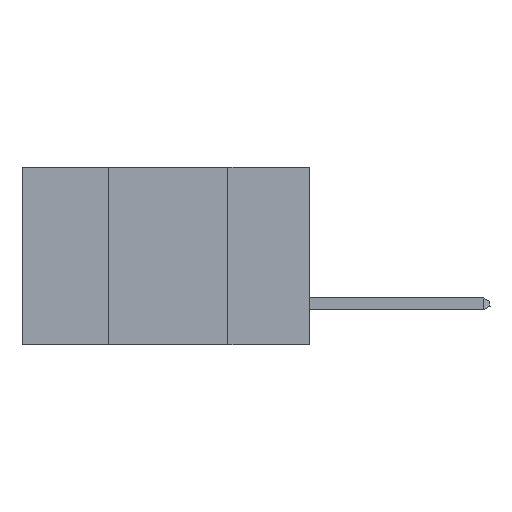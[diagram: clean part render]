
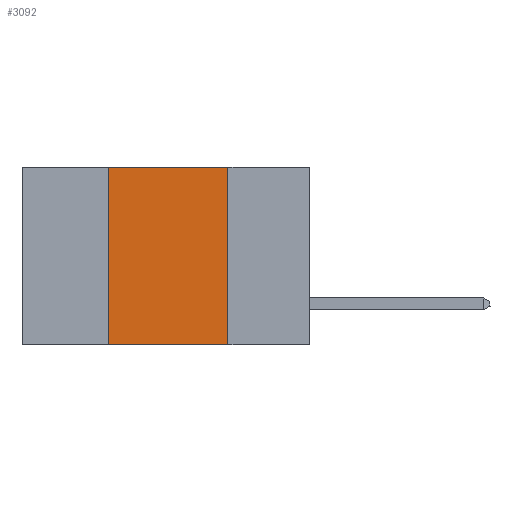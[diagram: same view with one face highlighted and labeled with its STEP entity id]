
A CAD part, left-side view. The second image highlights one B-rep face of the part: STEP entity #3092.
In plain terms, the highlighted planar face has unit normal (-1, 0, 0).
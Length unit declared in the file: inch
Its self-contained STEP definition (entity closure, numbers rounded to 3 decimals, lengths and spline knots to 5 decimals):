
#210 = CARTESIAN_POINT ( 'NONE',  ( 0., 0.42, 0. ) ) ;
#388 = LINE ( 'NONE', #210, #5888 ) ;
#428 = EDGE_CURVE ( 'NONE', #5441, #2898, #4499, .T. ) ;
#734 = CARTESIAN_POINT ( 'NONE',  ( 0., 0.42, 0. ) ) ;
#1393 = EDGE_LOOP ( 'NONE', ( #11305, #9578, #7424, #3486 ) ) ;
#2117 = AXIS2_PLACEMENT_3D ( 'NONE', #6378, #9193, #10298 ) ;
#2200 = VECTOR ( 'NONE', #3060, 39.37008 ) ;
#2898 = VERTEX_POINT ( 'NONE', #10344 ) ;
#2950 = DIRECTION ( 'NONE',  ( 0., -1., 0. ) ) ;
#3060 = DIRECTION ( 'NONE',  ( 0., -1., 0. ) ) ;
#3092 = ADVANCED_FACE ( 'NONE', ( #5071 ), #5305, .F. ) ;
#3486 = ORIENTED_EDGE ( 'NONE', *, *, #6404, .T. ) ;
#4111 = CARTESIAN_POINT ( 'NONE',  ( 0., 0.17, 0. ) ) ;
#4120 = VERTEX_POINT ( 'NONE', #8889 ) ;
#4499 = LINE ( 'NONE', #10944, #2200 ) ;
#4831 = VECTOR ( 'NONE', #2950, 39.37008 ) ;
#5071 = FACE_OUTER_BOUND ( 'NONE', #1393, .T. ) ;
#5305 = PLANE ( 'NONE',  #2117 ) ;
#5441 = VERTEX_POINT ( 'NONE', #734 ) ;
#5597 = LINE ( 'NONE', #4111, #6375 ) ;
#5888 = VECTOR ( 'NONE', #6737, 39.37008 ) ;
#6375 = VECTOR ( 'NONE', #10933, 39.37008 ) ;
#6378 = CARTESIAN_POINT ( 'NONE',  ( 0., 0.6, 0. ) ) ;
#6404 = EDGE_CURVE ( 'NONE', #11308, #4120, #11228, .T. ) ;
#6737 = DIRECTION ( 'NONE',  ( 0., 0., 1. ) ) ;
#7424 = ORIENTED_EDGE ( 'NONE', *, *, #12007, .F. ) ;
#7965 = CARTESIAN_POINT ( 'NONE',  ( 0., 0.42, -0.37 ) ) ;
#8747 = CARTESIAN_POINT ( 'NONE',  ( 0., 0.6, -0.37 ) ) ;
#8889 = CARTESIAN_POINT ( 'NONE',  ( 0., 0.17, -0.37 ) ) ;
#9193 = DIRECTION ( 'NONE',  ( 1., 0., 0. ) ) ;
#9578 = ORIENTED_EDGE ( 'NONE', *, *, #428, .F. ) ;
#10298 = DIRECTION ( 'NONE',  ( 0., 0., -1. ) ) ;
#10344 = CARTESIAN_POINT ( 'NONE',  ( 0., 0.17, 0. ) ) ;
#10933 = DIRECTION ( 'NONE',  ( 0., 0., -1. ) ) ;
#10944 = CARTESIAN_POINT ( 'NONE',  ( 0., 0.6, 0. ) ) ;
#11228 = LINE ( 'NONE', #8747, #4831 ) ;
#11305 = ORIENTED_EDGE ( 'NONE', *, *, #11327, .F. ) ;
#11308 = VERTEX_POINT ( 'NONE', #7965 ) ;
#11327 = EDGE_CURVE ( 'NONE', #2898, #4120, #5597, .T. ) ;
#12007 = EDGE_CURVE ( 'NONE', #11308, #5441, #388, .T. ) ;
